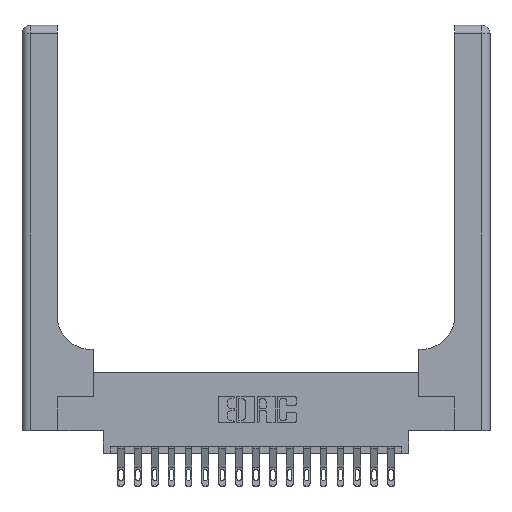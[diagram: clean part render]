
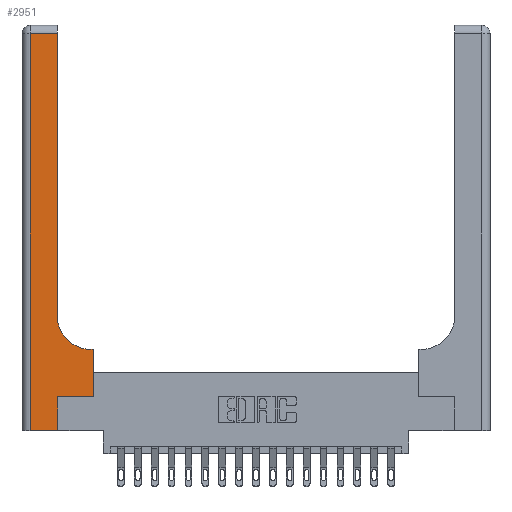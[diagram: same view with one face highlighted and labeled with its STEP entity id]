
A CAD part, top view. The second image highlights one B-rep face of the part: STEP entity #2951.
In plain terms, the highlighted planar face has unit normal (0, 0, 1).
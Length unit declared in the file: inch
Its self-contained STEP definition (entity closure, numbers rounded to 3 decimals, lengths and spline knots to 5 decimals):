
#238 = VERTEX_POINT ( 'NONE', #14843 ) ;
#354 = EDGE_CURVE ( 'NONE', #13176, #7606, #9215, .T. ) ;
#718 = VECTOR ( 'NONE', #15553, 39.37008 ) ;
#794 = VECTOR ( 'NONE', #13106, 39.37008 ) ;
#826 = CARTESIAN_POINT ( 'NONE',  ( 0., 2.94, 0.37 ) ) ;
#881 = ORIENTED_EDGE ( 'NONE', *, *, #16696, .T. ) ;
#1207 = CARTESIAN_POINT ( 'NONE',  ( 0.26, 0.6, 0.37 ) ) ;
#1399 = DIRECTION ( 'NONE',  ( 0., 1., 0. ) ) ;
#1581 = CARTESIAN_POINT ( 'NONE',  ( 0.51, 0.85, 0.37 ) ) ;
#1678 = VECTOR ( 'NONE', #15793, 39.37008 ) ;
#2195 = CARTESIAN_POINT ( 'NONE',  ( 0.26, 3., 0.37 ) ) ;
#2267 = DIRECTION ( 'NONE',  ( 0., 0., -1. ) ) ;
#2473 = DIRECTION ( 'NONE',  ( -1., 0., 0. ) ) ;
#2566 = VERTEX_POINT ( 'NONE', #10204 ) ;
#2725 = CIRCLE ( 'NONE', #5399, 0.25 ) ;
#2792 = VERTEX_POINT ( 'NONE', #6337 ) ;
#2825 = EDGE_CURVE ( 'NONE', #16898, #13176, #17650, .T. ) ;
#2951 = ADVANCED_FACE ( 'NONE', ( #11635 ), #14849, .F. ) ;
#3013 = DIRECTION ( 'NONE',  ( 1., 0., 0. ) ) ;
#3241 = DIRECTION ( 'NONE',  ( 0., 0., -1. ) ) ;
#3746 = CARTESIAN_POINT ( 'NONE',  ( 0.528, 0.6, 0.37 ) ) ;
#3875 = EDGE_CURVE ( 'NONE', #5416, #2792, #10206, .T. ) ;
#4792 = ORIENTED_EDGE ( 'NONE', *, *, #10095, .T. ) ;
#5399 = AXIS2_PLACEMENT_3D ( 'NONE', #1581, #3241, #12706 ) ;
#5400 = ORIENTED_EDGE ( 'NONE', *, *, #14463, .T. ) ;
#5416 = VERTEX_POINT ( 'NONE', #5578 ) ;
#5578 = CARTESIAN_POINT ( 'NONE',  ( 0.26, 2.94, 0.37 ) ) ;
#5704 = VECTOR ( 'NONE', #2473, 39.37008 ) ;
#5862 = VERTEX_POINT ( 'NONE', #18020 ) ;
#6202 = CARTESIAN_POINT ( 'NONE',  ( 0.528, 0.25, 0.37 ) ) ;
#6337 = CARTESIAN_POINT ( 'NONE',  ( 0.06, 2.94, 0.37 ) ) ;
#6440 = VECTOR ( 'NONE', #9762, 39.37008 ) ;
#6787 = DIRECTION ( 'NONE',  ( 0., 1., 0. ) ) ;
#7606 = VERTEX_POINT ( 'NONE', #3746 ) ;
#7906 = CARTESIAN_POINT ( 'NONE',  ( 0., 0., 0.37 ) ) ;
#9215 = LINE ( 'NONE', #18658, #718 ) ;
#9220 = EDGE_CURVE ( 'NONE', #2566, #5862, #15904, .T. ) ;
#9242 = ORIENTED_EDGE ( 'NONE', *, *, #3875, .T. ) ;
#9683 = VECTOR ( 'NONE', #6787, 39.37008 ) ;
#9762 = DIRECTION ( 'NONE',  ( 1., 0., 0. ) ) ;
#9858 = VECTOR ( 'NONE', #3013, 39.37008 ) ;
#9905 = VERTEX_POINT ( 'NONE', #12030 ) ;
#10095 = EDGE_CURVE ( 'NONE', #5862, #16898, #15642, .T. ) ;
#10204 = CARTESIAN_POINT ( 'NONE',  ( 0.06, 0., 0.37 ) ) ;
#10206 = LINE ( 'NONE', #826, #794 ) ;
#11635 = FACE_OUTER_BOUND ( 'NONE', #18975, .T. ) ;
#11811 = ORIENTED_EDGE ( 'NONE', *, *, #2825, .T. ) ;
#12030 = CARTESIAN_POINT ( 'NONE',  ( 0.51, 0.6, 0.37 ) ) ;
#12120 = ORIENTED_EDGE ( 'NONE', *, *, #9220, .T. ) ;
#12142 = LINE ( 'NONE', #1207, #5704 ) ;
#12427 = CARTESIAN_POINT ( 'NONE',  ( 0.265, 0., 0.37 ) ) ;
#12706 = DIRECTION ( 'NONE',  ( 1., 0., 0. ) ) ;
#12778 = CARTESIAN_POINT ( 'NONE',  ( 0.265, 0.25, 0.37 ) ) ;
#12907 = LINE ( 'NONE', #2195, #9683 ) ;
#13106 = DIRECTION ( 'NONE',  ( -1., 0., 0. ) ) ;
#13176 = VERTEX_POINT ( 'NONE', #6202 ) ;
#14145 = EDGE_CURVE ( 'NONE', #2792, #2566, #17447, .T. ) ;
#14463 = EDGE_CURVE ( 'NONE', #7606, #9905, #12142, .T. ) ;
#14843 = CARTESIAN_POINT ( 'NONE',  ( 0.26, 0.85, 0.37 ) ) ;
#14849 = PLANE ( 'NONE',  #18701 ) ;
#15553 = DIRECTION ( 'NONE',  ( 0., 1., 0. ) ) ;
#15642 = LINE ( 'NONE', #12427, #18506 ) ;
#15793 = DIRECTION ( 'NONE',  ( 0., -1., 0. ) ) ;
#15904 = LINE ( 'NONE', #7906, #9858 ) ;
#15986 = ORIENTED_EDGE ( 'NONE', *, *, #354, .T. ) ;
#16696 = EDGE_CURVE ( 'NONE', #238, #5416, #12907, .T. ) ;
#16898 = VERTEX_POINT ( 'NONE', #19849 ) ;
#16948 = EDGE_CURVE ( 'NONE', #9905, #238, #2725, .T. ) ;
#17447 = LINE ( 'NONE', #19099, #1678 ) ;
#17484 = ORIENTED_EDGE ( 'NONE', *, *, #16948, .T. ) ;
#17650 = LINE ( 'NONE', #12778, #6440 ) ;
#17870 = ORIENTED_EDGE ( 'NONE', *, *, #14145, .T. ) ;
#17959 = DIRECTION ( 'NONE',  ( -1., 0., 0. ) ) ;
#18020 = CARTESIAN_POINT ( 'NONE',  ( 0.265, 0., 0.37 ) ) ;
#18066 = CARTESIAN_POINT ( 'NONE',  ( 0., 3., 0.37 ) ) ;
#18506 = VECTOR ( 'NONE', #1399, 39.37008 ) ;
#18658 = CARTESIAN_POINT ( 'NONE',  ( 0.528, 0.25, 0.37 ) ) ;
#18701 = AXIS2_PLACEMENT_3D ( 'NONE', #18066, #2267, #17959 ) ;
#18975 = EDGE_LOOP ( 'NONE', ( #881, #9242, #17870, #12120, #4792, #11811, #15986, #5400, #17484 ) ) ;
#19099 = CARTESIAN_POINT ( 'NONE',  ( 0.06, 3., 0.37 ) ) ;
#19849 = CARTESIAN_POINT ( 'NONE',  ( 0.265, 0.25, 0.37 ) ) ;
